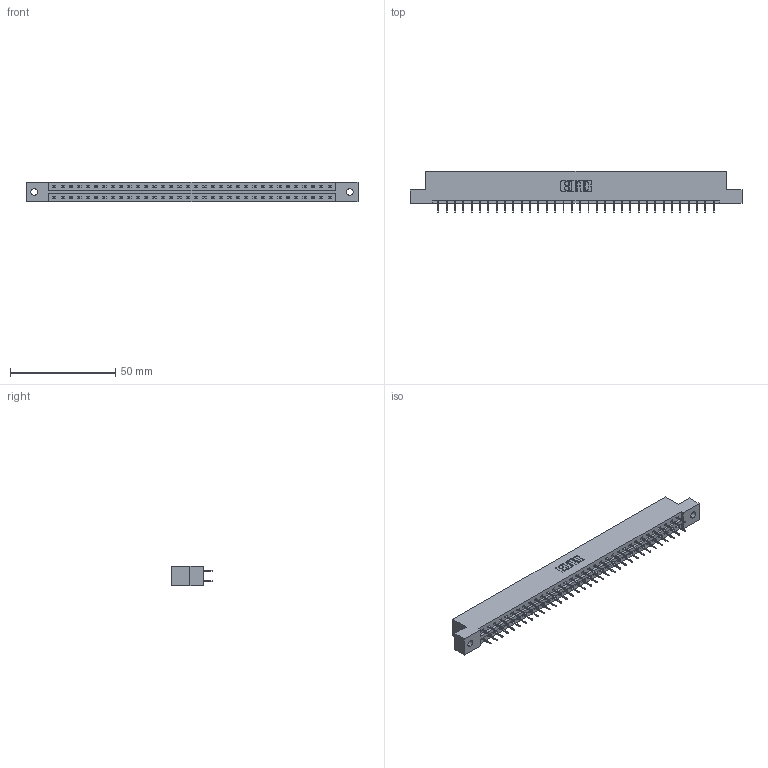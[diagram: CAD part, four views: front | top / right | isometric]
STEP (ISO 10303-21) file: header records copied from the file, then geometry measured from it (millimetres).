
FILE_DESCRIPTION (( 'STEP AP203' ), '1' );
FILE_NAME ('337-068-524-202.STEP', '2018-08-11T09:42:29', ( '' ), ( '' ), 'SwSTEP 2.0', 'SolidWorks 2016', '' );
FILE_SCHEMA (( 'CONFIG_CONTROL_DESIGN' ));
Length unit declared in the file: inch
Products named in the file (3): 337 Part_Flush Mounting Lugs - 0.128 Dia; 345-292-001_345-293-124; 337-068-524-202
Assembly tree (69 placements, depth 2):
  337-068-524-202
    337 Part_Flush Mounting Lugs - 0.128 Dia
    345-292-001_345-293-124  x68
Bounding box: 157.73 x 19.69 x 9.4 mm (x, y, z)
Volume: 16377.2 mm3; surface area: 17845.3 mm2
Topology: 69 solids, 69 shells, 4058 faces, 11531 edges, 7414 vertices
Faces by surface type: plane 3062, cylinder 996
Entity records: 27473 total; most frequent: CARTESIAN_POINT 4634, ORIENTED_EDGE 4570, DIRECTION 3957, EDGE_CURVE 2285, VECTOR 2161, LINE 2161, VERTEX_POINT 1518, AXIS2_PLACEMENT_3D 898
